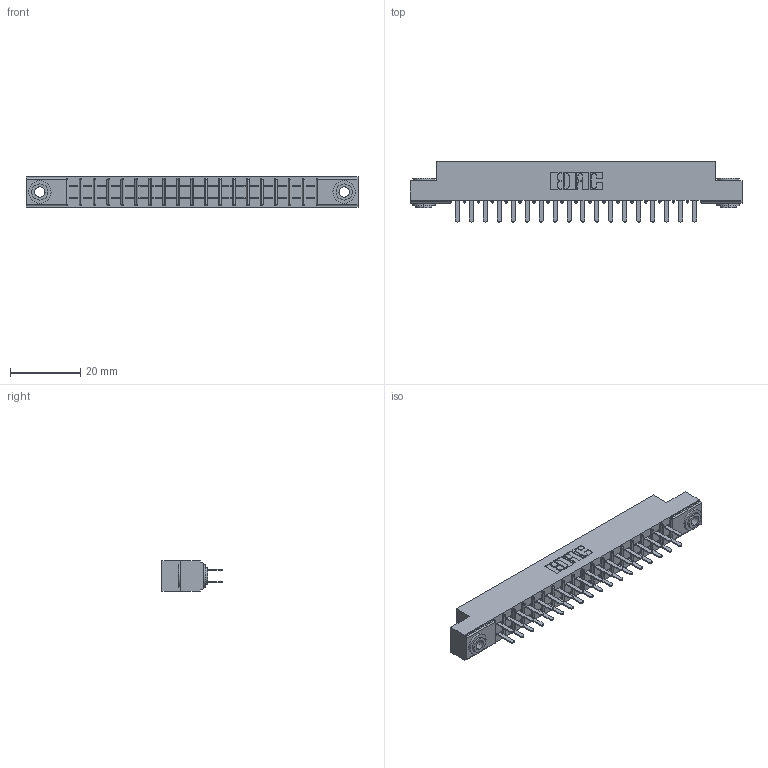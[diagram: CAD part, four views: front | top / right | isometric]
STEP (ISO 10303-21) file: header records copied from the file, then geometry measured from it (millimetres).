
FILE_DESCRIPTION (( 'STEP AP203' ), '1' );
FILE_NAME ('355-036-520-503.STEP', '2019-09-11T09:30:58', ( '' ), ( '' ), 'SwSTEP 2.0', 'SolidWorks 2016', '' );
FILE_SCHEMA (( 'CONFIG_CONTROL_DESIGN' ));
Length unit declared in the file: inch
Products named in the file (4): 355-036-520-503; 305-290-001_520; 345-250-002_345-250-002-102; 305 Part_.156 Dia
Assembly tree (39 placements, depth 2):
  355-036-520-503
    305 Part_.156 Dia
    305-290-001_520  x36
    345-250-002_345-250-002-102  x2
Bounding box: 94.34 x 17.09 x 8.71 mm (x, y, z)
Volume: 5667.1 mm3; surface area: 11309.2 mm2
Topology: 39 solids, 39 shells, 1824 faces, 5162 edges, 3340 vertices
Faces by surface type: plane 1064, cylinder 680, sphere 72, cone 8
Entity records: 23356 total; most frequent: CARTESIAN_POINT 3845, ORIENTED_EDGE 3804, DIRECTION 3754, EDGE_CURVE 1902, VECTOR 1504, LINE 1504, VERTEX_POINT 1216, AXIS2_PLACEMENT_3D 1125
